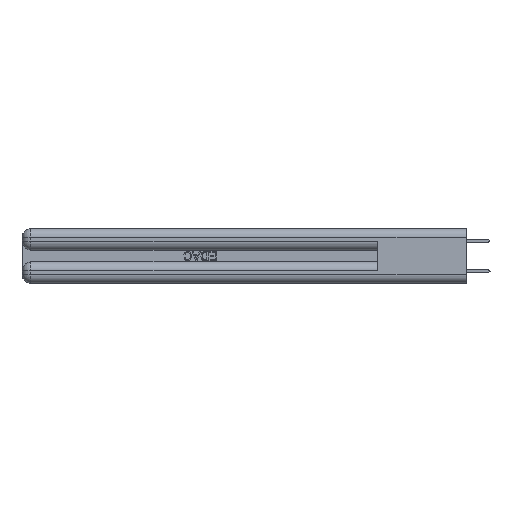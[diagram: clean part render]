
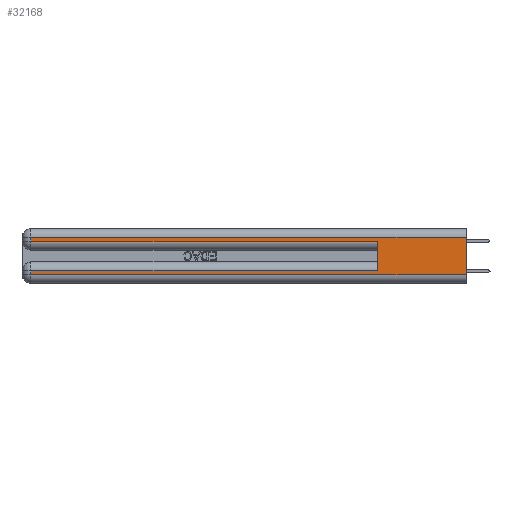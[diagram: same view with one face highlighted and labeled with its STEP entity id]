
A CAD part, left-side view. The second image highlights one B-rep face of the part: STEP entity #32168.
In plain terms, the highlighted planar face has unit normal (-1, 0, 0).
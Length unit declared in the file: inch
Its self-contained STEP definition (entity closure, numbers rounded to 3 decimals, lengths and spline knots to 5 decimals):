
#493 = VERTEX_POINT ( 'NONE', #6584 ) ;
#1935 = DIRECTION ( 'NONE',  ( 0., 0., 1. ) ) ;
#1978 = VECTOR ( 'NONE', #3143, 39.37008 ) ;
#2075 = EDGE_CURVE ( 'NONE', #30776, #5658, #10205, .T. ) ;
#2270 = ORIENTED_EDGE ( 'NONE', *, *, #30695, .F. ) ;
#3143 = DIRECTION ( 'NONE',  ( 0., 1., 0. ) ) ;
#3798 = ORIENTED_EDGE ( 'NONE', *, *, #24242, .T. ) ;
#4291 = DIRECTION ( 'NONE',  ( 0., -1., 0. ) ) ;
#5366 = CARTESIAN_POINT ( 'NONE',  ( 0., 0., 0.06 ) ) ;
#5384 = VERTEX_POINT ( 'NONE', #27377 ) ;
#5395 = VECTOR ( 'NONE', #10307, 39.37008 ) ;
#5658 = VERTEX_POINT ( 'NONE', #5366 ) ;
#6501 = VERTEX_POINT ( 'NONE', #23709 ) ;
#6584 = CARTESIAN_POINT ( 'NONE',  ( 0., 2.94, 0.06 ) ) ;
#8319 = ORIENTED_EDGE ( 'NONE', *, *, #26705, .T. ) ;
#8337 = EDGE_LOOP ( 'NONE', ( #16905, #23349, #3798, #8319, #2270, #10006, #40976, #28692 ) ) ;
#8578 = CARTESIAN_POINT ( 'NONE',  ( 0., 0.6, 0.285 ) ) ;
#9153 = VECTOR ( 'NONE', #36024, 39.37008 ) ;
#9482 = FACE_OUTER_BOUND ( 'NONE', #8337, .T. ) ;
#10006 = ORIENTED_EDGE ( 'NONE', *, *, #37639, .T. ) ;
#10205 = LINE ( 'NONE', #42621, #9153 ) ;
#10307 = DIRECTION ( 'NONE',  ( 0., 0., -1. ) ) ;
#10608 = CARTESIAN_POINT ( 'NONE',  ( 0., 2.94, 0.31 ) ) ;
#11125 = CARTESIAN_POINT ( 'NONE',  ( 0., 2.94, 0.37 ) ) ;
#11712 = LINE ( 'NONE', #18350, #30066 ) ;
#13008 = LINE ( 'NONE', #33233, #1978 ) ;
#13611 = LINE ( 'NONE', #29271, #24056 ) ;
#14280 = CARTESIAN_POINT ( 'NONE',  ( 0., 0., 0.06 ) ) ;
#14790 = EDGE_CURVE ( 'NONE', #30776, #16148, #13008, .T. ) ;
#15619 = DIRECTION ( 'NONE',  ( 0., 1., 0. ) ) ;
#16148 = VERTEX_POINT ( 'NONE', #10608 ) ;
#16378 = LINE ( 'NONE', #14280, #23177 ) ;
#16905 = ORIENTED_EDGE ( 'NONE', *, *, #2075, .F. ) ;
#16934 = LINE ( 'NONE', #20801, #5395 ) ;
#18274 = VERTEX_POINT ( 'NONE', #18862 ) ;
#18350 = CARTESIAN_POINT ( 'NONE',  ( 0., 0.6, 0.145 ) ) ;
#18862 = CARTESIAN_POINT ( 'NONE',  ( 0., 2.94, 0.085 ) ) ;
#20801 = CARTESIAN_POINT ( 'NONE',  ( 0., 2.94, 0.37 ) ) ;
#23177 = VECTOR ( 'NONE', #4291, 39.37008 ) ;
#23349 = ORIENTED_EDGE ( 'NONE', *, *, #14790, .T. ) ;
#23361 = DIRECTION ( 'NONE',  ( 0., 0., -1. ) ) ;
#23709 = CARTESIAN_POINT ( 'NONE',  ( 0., 2.94, 0.285 ) ) ;
#24039 = DIRECTION ( 'NONE',  ( 0., -1., 0. ) ) ;
#24056 = VECTOR ( 'NONE', #15619, 39.37008 ) ;
#24242 = EDGE_CURVE ( 'NONE', #16148, #6501, #16934, .T. ) ;
#24421 = DIRECTION ( 'NONE',  ( 0., 0., -1. ) ) ;
#24484 = EDGE_CURVE ( 'NONE', #493, #5658, #16378, .T. ) ;
#25962 = VECTOR ( 'NONE', #24421, 39.37008 ) ;
#26705 = EDGE_CURVE ( 'NONE', #6501, #40755, #29331, .T. ) ;
#26733 = CARTESIAN_POINT ( 'NONE',  ( 0., 0., 0.37 ) ) ;
#27018 = LINE ( 'NONE', #11125, #25962 ) ;
#27377 = CARTESIAN_POINT ( 'NONE',  ( 0., 0.6, 0.085 ) ) ;
#28582 = AXIS2_PLACEMENT_3D ( 'NONE', #26733, #30160, #23361 ) ;
#28692 = ORIENTED_EDGE ( 'NONE', *, *, #24484, .T. ) ;
#29271 = CARTESIAN_POINT ( 'NONE',  ( 0., 0., 0.085 ) ) ;
#29331 = LINE ( 'NONE', #29818, #41893 ) ;
#29818 = CARTESIAN_POINT ( 'NONE',  ( 0., 0., 0.285 ) ) ;
#30066 = VECTOR ( 'NONE', #1935, 39.37008 ) ;
#30160 = DIRECTION ( 'NONE',  ( 1., 0., 0. ) ) ;
#30695 = EDGE_CURVE ( 'NONE', #5384, #40755, #11712, .T. ) ;
#30776 = VERTEX_POINT ( 'NONE', #35539 ) ;
#32168 = ADVANCED_FACE ( 'NONE', ( #9482 ), #33697, .F. ) ;
#33233 = CARTESIAN_POINT ( 'NONE',  ( 0., 0., 0.31 ) ) ;
#33697 = PLANE ( 'NONE',  #28582 ) ;
#34213 = EDGE_CURVE ( 'NONE', #18274, #493, #27018, .T. ) ;
#35539 = CARTESIAN_POINT ( 'NONE',  ( 0., 0., 0.31 ) ) ;
#36024 = DIRECTION ( 'NONE',  ( 0., 0., -1. ) ) ;
#37639 = EDGE_CURVE ( 'NONE', #5384, #18274, #13611, .T. ) ;
#40755 = VERTEX_POINT ( 'NONE', #8578 ) ;
#40976 = ORIENTED_EDGE ( 'NONE', *, *, #34213, .T. ) ;
#41893 = VECTOR ( 'NONE', #24039, 39.37008 ) ;
#42621 = CARTESIAN_POINT ( 'NONE',  ( 0., 0., 0.37 ) ) ;
